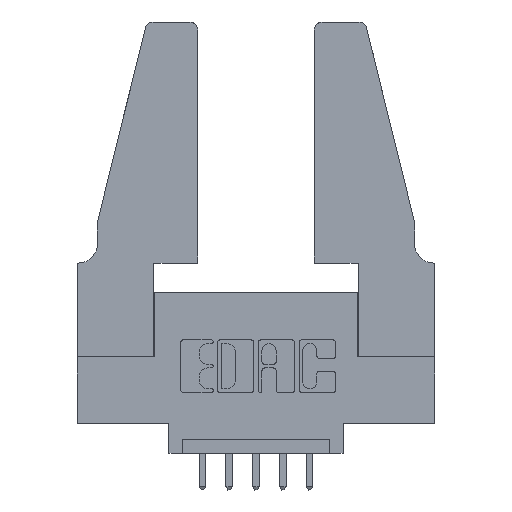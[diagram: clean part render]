
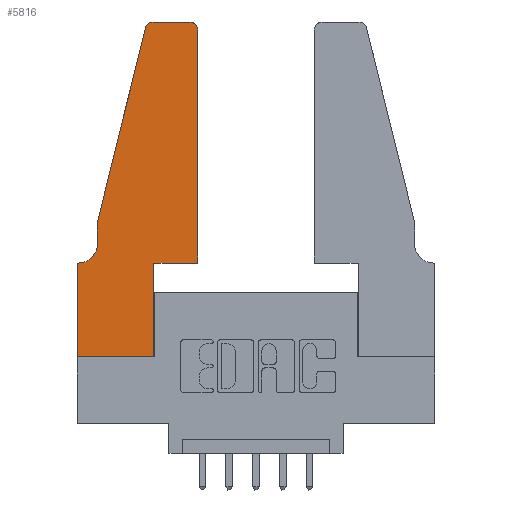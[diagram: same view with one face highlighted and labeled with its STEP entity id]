
A CAD part, top view. The second image highlights one B-rep face of the part: STEP entity #5816.
In plain terms, the highlighted planar face has unit normal (0, 0, 1).
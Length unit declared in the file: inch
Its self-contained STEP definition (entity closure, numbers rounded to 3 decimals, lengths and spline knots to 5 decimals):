
#101 = DIRECTION ( 'NONE',  ( 0., 1., 0. ) ) ;
#241 = DIRECTION ( 'NONE',  ( -1., 0., 0. ) ) ;
#293 = EDGE_CURVE ( 'NONE', #4091, #9027, #1606, .T. ) ;
#335 = EDGE_CURVE ( 'NONE', #9689, #8200, #664, .T. ) ;
#364 = DIRECTION ( 'NONE',  ( 0., 1., 0. ) ) ;
#664 = LINE ( 'NONE', #3756, #7069 ) ;
#753 = CARTESIAN_POINT ( 'NONE',  ( 0.2865, 0., 0.37 ) ) ;
#761 = DIRECTION ( 'NONE',  ( -0.239, -0.971, 0. ) ) ;
#767 = VERTEX_POINT ( 'NONE', #6638 ) ;
#798 = LINE ( 'NONE', #10539, #10433 ) ;
#960 = DIRECTION ( 'NONE',  ( 0., 0., 1. ) ) ;
#986 = DIRECTION ( 'NONE',  ( 0., 0., -1. ) ) ;
#1031 = LINE ( 'NONE', #10214, #5321 ) ;
#1117 = DIRECTION ( 'NONE',  ( 1., 0., 0. ) ) ;
#1153 = LINE ( 'NONE', #7903, #7163 ) ;
#1190 = ORIENTED_EDGE ( 'NONE', *, *, #5367, .T. ) ;
#1546 = CARTESIAN_POINT ( 'NONE',  ( 0., 0., 0.37 ) ) ;
#1606 = LINE ( 'NONE', #6233, #8147 ) ;
#1633 = ORIENTED_EDGE ( 'NONE', *, *, #4875, .T. ) ;
#1824 = VECTOR ( 'NONE', #101, 39.37008 ) ;
#1999 = FACE_OUTER_BOUND ( 'NONE', #7382, .T. ) ;
#2161 = CARTESIAN_POINT ( 'NONE',  ( 0.25487, 1.22718, 0.37 ) ) ;
#2169 = AXIS2_PLACEMENT_3D ( 'NONE', #2349, #9091, #4061 ) ;
#2292 = EDGE_CURVE ( 'NONE', #6300, #767, #1031, .T. ) ;
#2312 = ORIENTED_EDGE ( 'NONE', *, *, #335, .T. ) ;
#2349 = CARTESIAN_POINT ( 'NONE',  ( 0., 0.35, 0.37 ) ) ;
#2354 = EDGE_CURVE ( 'NONE', #5677, #5262, #9567, .T. ) ;
#2708 = CARTESIAN_POINT ( 'NONE',  ( 0.4205, 1.22, 0.37 ) ) ;
#2880 = CARTESIAN_POINT ( 'NONE',  ( 0., 0.35, 0.37 ) ) ;
#2930 = ORIENTED_EDGE ( 'NONE', *, *, #6779, .T. ) ;
#3036 = EDGE_CURVE ( 'NONE', #5262, #8943, #1153, .T. ) ;
#3213 = CARTESIAN_POINT ( 'NONE',  ( 0.0755, 0.5, 0.37 ) ) ;
#3431 = CARTESIAN_POINT ( 'NONE',  ( 0.0755, 0.5, 0.37 ) ) ;
#3545 = ORIENTED_EDGE ( 'NONE', *, *, #2354, .T. ) ;
#3654 = ORIENTED_EDGE ( 'NONE', *, *, #4574, .T. ) ;
#3756 = CARTESIAN_POINT ( 'NONE',  ( 0., 0., 0.37 ) ) ;
#3953 = VERTEX_POINT ( 'NONE', #8488 ) ;
#3992 = VECTOR ( 'NONE', #5851, 39.37008 ) ;
#4061 = DIRECTION ( 'NONE',  ( 1., 0., 0. ) ) ;
#4091 = VERTEX_POINT ( 'NONE', #6768 ) ;
#4235 = CIRCLE ( 'NONE', #9284, 0.03 ) ;
#4306 = LINE ( 'NONE', #10060, #5368 ) ;
#4327 = ORIENTED_EDGE ( 'NONE', *, *, #293, .T. ) ;
#4345 = DIRECTION ( 'NONE',  ( 1., 0., 0. ) ) ;
#4574 = EDGE_CURVE ( 'NONE', #5397, #6934, #4306, .T. ) ;
#4771 = PLANE ( 'NONE',  #2169 ) ;
#4809 = DIRECTION ( 'NONE',  ( 1., 0., 0. ) ) ;
#4875 = EDGE_CURVE ( 'NONE', #8200, #4091, #798, .T. ) ;
#5262 = VERTEX_POINT ( 'NONE', #8884 ) ;
#5321 = VECTOR ( 'NONE', #7677, 39.37008 ) ;
#5367 = EDGE_CURVE ( 'NONE', #767, #5397, #6933, .T. ) ;
#5368 = VECTOR ( 'NONE', #761, 39.37008 ) ;
#5388 = DIRECTION ( 'NONE',  ( 1., 0., 0. ) ) ;
#5397 = VERTEX_POINT ( 'NONE', #2161 ) ;
#5662 = DIRECTION ( 'NONE',  ( 0., 0., 1. ) ) ;
#5677 = VERTEX_POINT ( 'NONE', #8761 ) ;
#5816 = ADVANCED_FACE ( 'NONE', ( #1999 ), #4771, .T. ) ;
#5851 = DIRECTION ( 'NONE',  ( 0., -1., 0. ) ) ;
#5985 = LINE ( 'NONE', #6720, #7974 ) ;
#6034 = ORIENTED_EDGE ( 'NONE', *, *, #3036, .T. ) ;
#6086 = LINE ( 'NONE', #6870, #1824 ) ;
#6233 = CARTESIAN_POINT ( 'NONE',  ( 0.4505, 0.35, 0.37 ) ) ;
#6300 = VERTEX_POINT ( 'NONE', #10761 ) ;
#6584 = EDGE_CURVE ( 'NONE', #8943, #9689, #5985, .T. ) ;
#6638 = CARTESIAN_POINT ( 'NONE',  ( 0.284, 1.25, 0.37 ) ) ;
#6720 = CARTESIAN_POINT ( 'NONE',  ( 0., 0., 0.37 ) ) ;
#6758 = DIRECTION ( 'NONE',  ( 0., -1., 0. ) ) ;
#6768 = CARTESIAN_POINT ( 'NONE',  ( 0.2865, 0.35, 0.37 ) ) ;
#6779 = EDGE_CURVE ( 'NONE', #6934, #5677, #10245, .T. ) ;
#6870 = CARTESIAN_POINT ( 'NONE',  ( 0.4505, 0.35, 0.37 ) ) ;
#6933 = CIRCLE ( 'NONE', #7142, 0.03 ) ;
#6934 = VERTEX_POINT ( 'NONE', #3431 ) ;
#7069 = VECTOR ( 'NONE', #1117, 39.37008 ) ;
#7142 = AXIS2_PLACEMENT_3D ( 'NONE', #7324, #5662, #4809 ) ;
#7163 = VECTOR ( 'NONE', #8743, 39.37008 ) ;
#7324 = CARTESIAN_POINT ( 'NONE',  ( 0.284, 1.22, 0.37 ) ) ;
#7365 = EDGE_CURVE ( 'NONE', #3953, #6300, #4235, .T. ) ;
#7367 = EDGE_CURVE ( 'NONE', #9027, #3953, #6086, .T. ) ;
#7382 = EDGE_LOOP ( 'NONE', ( #11012, #1190, #3654, #2930, #3545, #6034, #7732, #2312, #1633, #4327, #9129, #10082 ) ) ;
#7486 = CARTESIAN_POINT ( 'NONE',  ( 0.4505, 0.35, 0.37 ) ) ;
#7677 = DIRECTION ( 'NONE',  ( -1., 0., 0. ) ) ;
#7732 = ORIENTED_EDGE ( 'NONE', *, *, #6584, .T. ) ;
#7783 = CARTESIAN_POINT ( 'NONE',  ( 0.0055, 0.42, 0.37 ) ) ;
#7903 = CARTESIAN_POINT ( 'NONE',  ( 0.0755, 0.35, 0.37 ) ) ;
#7974 = VECTOR ( 'NONE', #6758, 39.37008 ) ;
#8147 = VECTOR ( 'NONE', #5388, 39.37008 ) ;
#8200 = VERTEX_POINT ( 'NONE', #753 ) ;
#8488 = CARTESIAN_POINT ( 'NONE',  ( 0.4505, 1.22, 0.37 ) ) ;
#8743 = DIRECTION ( 'NONE',  ( -1., 0., 0. ) ) ;
#8761 = CARTESIAN_POINT ( 'NONE',  ( 0.0755, 0.42, 0.37 ) ) ;
#8884 = CARTESIAN_POINT ( 'NONE',  ( 0.0055, 0.35, 0.37 ) ) ;
#8943 = VERTEX_POINT ( 'NONE', #2880 ) ;
#9027 = VERTEX_POINT ( 'NONE', #7486 ) ;
#9091 = DIRECTION ( 'NONE',  ( 0., 0., 1. ) ) ;
#9129 = ORIENTED_EDGE ( 'NONE', *, *, #7367, .T. ) ;
#9284 = AXIS2_PLACEMENT_3D ( 'NONE', #2708, #960, #4345 ) ;
#9467 = AXIS2_PLACEMENT_3D ( 'NONE', #7783, #986, #241 ) ;
#9567 = CIRCLE ( 'NONE', #9467, 0.07 ) ;
#9689 = VERTEX_POINT ( 'NONE', #1546 ) ;
#10060 = CARTESIAN_POINT ( 'NONE',  ( 0.0755, 0.5, 0.37 ) ) ;
#10082 = ORIENTED_EDGE ( 'NONE', *, *, #7365, .T. ) ;
#10214 = CARTESIAN_POINT ( 'NONE',  ( 0.2605, 1.25, 0.37 ) ) ;
#10245 = LINE ( 'NONE', #3213, #3992 ) ;
#10433 = VECTOR ( 'NONE', #364, 39.37008 ) ;
#10539 = CARTESIAN_POINT ( 'NONE',  ( 0.2865, 0.35, 0.37 ) ) ;
#10761 = CARTESIAN_POINT ( 'NONE',  ( 0.4205, 1.25, 0.37 ) ) ;
#11012 = ORIENTED_EDGE ( 'NONE', *, *, #2292, .T. ) ;
